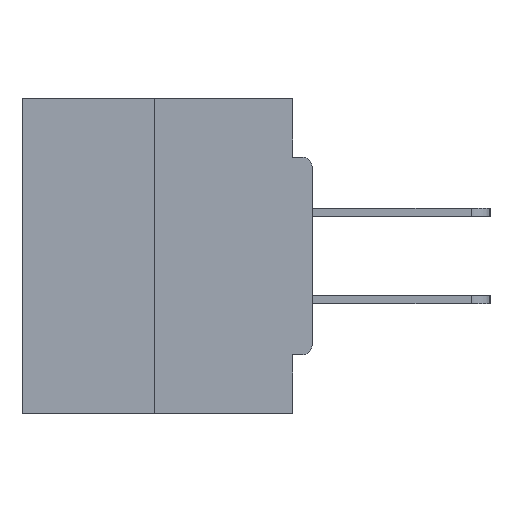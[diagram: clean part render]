
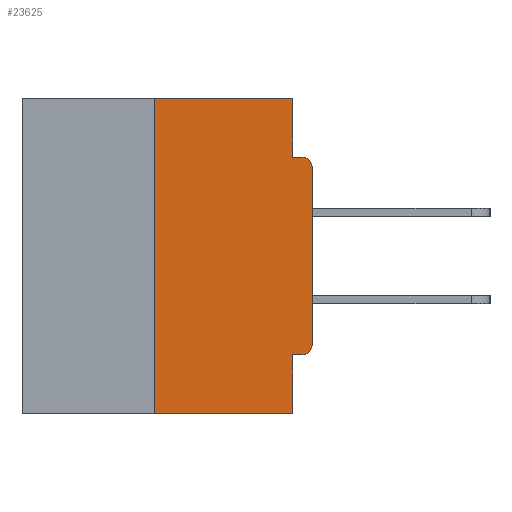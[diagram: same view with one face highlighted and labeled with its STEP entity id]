
A CAD part, left-side view. The second image highlights one B-rep face of the part: STEP entity #23625.
In plain terms, the highlighted planar face has unit normal (-1, 0, 0).
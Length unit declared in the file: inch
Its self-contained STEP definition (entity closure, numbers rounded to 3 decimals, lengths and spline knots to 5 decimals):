
#316 = CARTESIAN_POINT ( 'NONE',  ( 0., 0.25, -0.5 ) ) ;
#655 = VERTEX_POINT ( 'NONE', #3906 ) ;
#974 = LINE ( 'NONE', #31194, #27800 ) ;
#1180 = CARTESIAN_POINT ( 'NONE',  ( 0., 0.031, -0.4065 ) ) ;
#1892 = EDGE_CURVE ( 'NONE', #20515, #12876, #974, .T. ) ;
#2177 = DIRECTION ( 'NONE',  ( -1., 0., 0. ) ) ;
#2508 = CARTESIAN_POINT ( 'NONE',  ( 0., 0.015, -0.1085 ) ) ;
#3137 = LINE ( 'NONE', #16115, #3894 ) ;
#3481 = DIRECTION ( 'NONE',  ( 0., -1., 0. ) ) ;
#3575 = ORIENTED_EDGE ( 'NONE', *, *, #23578, .F. ) ;
#3604 = ORIENTED_EDGE ( 'NONE', *, *, #12128, .F. ) ;
#3894 = VECTOR ( 'NONE', #20548, 39.37008 ) ;
#3906 = CARTESIAN_POINT ( 'NONE',  ( 0., 0.015, -0.0935 ) ) ;
#4278 = DIRECTION ( 'NONE',  ( 0., 0., -1. ) ) ;
#4534 = VERTEX_POINT ( 'NONE', #9252 ) ;
#4629 = DIRECTION ( 'NONE',  ( 0., 0., 1. ) ) ;
#4662 = EDGE_CURVE ( 'NONE', #26802, #655, #10430, .T. ) ;
#4666 = CARTESIAN_POINT ( 'NONE',  ( 0., 0.031, 0. ) ) ;
#5532 = ORIENTED_EDGE ( 'NONE', *, *, #17376, .F. ) ;
#5582 = VERTEX_POINT ( 'NONE', #21843 ) ;
#5725 = CARTESIAN_POINT ( 'NONE',  ( 0., 0., -0.3915 ) ) ;
#5882 = DIRECTION ( 'NONE',  ( 0., 1., 0. ) ) ;
#6043 = DIRECTION ( 'NONE',  ( -1., 0., 0. ) ) ;
#6795 = ORIENTED_EDGE ( 'NONE', *, *, #1892, .F. ) ;
#7691 = EDGE_CURVE ( 'NONE', #27139, #26802, #31581, .T. ) ;
#8728 = CARTESIAN_POINT ( 'NONE',  ( 0., 0.46, 0. ) ) ;
#8793 = CARTESIAN_POINT ( 'NONE',  ( 0., 0.015, -0.4065 ) ) ;
#9252 = CARTESIAN_POINT ( 'NONE',  ( 0., 0.031, -0.0935 ) ) ;
#9364 = LINE ( 'NONE', #19391, #10899 ) ;
#9712 = AXIS2_PLACEMENT_3D ( 'NONE', #23467, #6043, #16069 ) ;
#9913 = CARTESIAN_POINT ( 'NONE',  ( 0., 0.031, 0. ) ) ;
#10430 = CIRCLE ( 'NONE', #30918, 0.015 ) ;
#10448 = CARTESIAN_POINT ( 'NONE',  ( 0., 0.031, -0.5 ) ) ;
#10782 = VERTEX_POINT ( 'NONE', #4666 ) ;
#10874 = VECTOR ( 'NONE', #19602, 39.37008 ) ;
#10899 = VECTOR ( 'NONE', #29411, 39.37008 ) ;
#11346 = CARTESIAN_POINT ( 'NONE',  ( 0., 0.46, 0. ) ) ;
#12128 = EDGE_CURVE ( 'NONE', #23002, #5582, #22257, .T. ) ;
#12876 = VERTEX_POINT ( 'NONE', #1180 ) ;
#16069 = DIRECTION ( 'NONE',  ( 0., 0., -1. ) ) ;
#16115 = CARTESIAN_POINT ( 'NONE',  ( 0., 0., -0.0935 ) ) ;
#16606 = VECTOR ( 'NONE', #3481, 39.37008 ) ;
#17376 = EDGE_CURVE ( 'NONE', #5582, #10782, #19076, .T. ) ;
#17404 = ORIENTED_EDGE ( 'NONE', *, *, #4662, .T. ) ;
#18247 = ORIENTED_EDGE ( 'NONE', *, *, #7691, .T. ) ;
#18555 = EDGE_LOOP ( 'NONE', ( #5532, #3604, #29578, #3575, #6795, #25475, #18247, #17404, #24689, #27252 ) ) ;
#18741 = EDGE_CURVE ( 'NONE', #20515, #27139, #23890, .T. ) ;
#18760 = PLANE ( 'NONE',  #28768 ) ;
#18796 = LINE ( 'NONE', #19420, #30150 ) ;
#19076 = LINE ( 'NONE', #8728, #16606 ) ;
#19230 = FACE_OUTER_BOUND ( 'NONE', #18555, .T. ) ;
#19391 = CARTESIAN_POINT ( 'NONE',  ( 0., 0.031, -0.5 ) ) ;
#19420 = CARTESIAN_POINT ( 'NONE',  ( 0., 0.46, -0.5 ) ) ;
#19602 = DIRECTION ( 'NONE',  ( 0., 0., -1. ) ) ;
#20515 = VERTEX_POINT ( 'NONE', #8793 ) ;
#20548 = DIRECTION ( 'NONE',  ( 0., -1., 0. ) ) ;
#20625 = EDGE_CURVE ( 'NONE', #10782, #4534, #32255, .T. ) ;
#21574 = CARTESIAN_POINT ( 'NONE',  ( 0., 0., 0. ) ) ;
#21580 = DIRECTION ( 'NONE',  ( 0., -1., 0. ) ) ;
#21843 = CARTESIAN_POINT ( 'NONE',  ( 0., 0.25, 0. ) ) ;
#22018 = DIRECTION ( 'NONE',  ( 1., 0., 0. ) ) ;
#22234 = VECTOR ( 'NONE', #31807, 39.37008 ) ;
#22257 = LINE ( 'NONE', #32276, #22234 ) ;
#23002 = VERTEX_POINT ( 'NONE', #316 ) ;
#23467 = CARTESIAN_POINT ( 'NONE',  ( 0., 0.015, -0.3915 ) ) ;
#23578 = EDGE_CURVE ( 'NONE', #12876, #32240, #9364, .T. ) ;
#23625 = ADVANCED_FACE ( 'NONE', ( #19230 ), #18760, .F. ) ;
#23663 = CARTESIAN_POINT ( 'NONE',  ( 0., 0., -0.1085 ) ) ;
#23890 = CIRCLE ( 'NONE', #9712, 0.015 ) ;
#24689 = ORIENTED_EDGE ( 'NONE', *, *, #28643, .F. ) ;
#24690 = DIRECTION ( 'NONE',  ( 0., 0., -1. ) ) ;
#25475 = ORIENTED_EDGE ( 'NONE', *, *, #18741, .T. ) ;
#26802 = VERTEX_POINT ( 'NONE', #23663 ) ;
#27139 = VERTEX_POINT ( 'NONE', #5725 ) ;
#27252 = ORIENTED_EDGE ( 'NONE', *, *, #20625, .F. ) ;
#27800 = VECTOR ( 'NONE', #5882, 39.37008 ) ;
#28643 = EDGE_CURVE ( 'NONE', #4534, #655, #3137, .T. ) ;
#28768 = AXIS2_PLACEMENT_3D ( 'NONE', #11346, #22018, #4278 ) ;
#29411 = DIRECTION ( 'NONE',  ( 0., 0., -1. ) ) ;
#29578 = ORIENTED_EDGE ( 'NONE', *, *, #29597, .T. ) ;
#29597 = EDGE_CURVE ( 'NONE', #23002, #32240, #18796, .T. ) ;
#30040 = VECTOR ( 'NONE', #4629, 39.37008 ) ;
#30150 = VECTOR ( 'NONE', #21580, 39.37008 ) ;
#30918 = AXIS2_PLACEMENT_3D ( 'NONE', #2508, #2177, #24690 ) ;
#31194 = CARTESIAN_POINT ( 'NONE',  ( 0., 0., -0.4065 ) ) ;
#31581 = LINE ( 'NONE', #21574, #30040 ) ;
#31807 = DIRECTION ( 'NONE',  ( 0., 0., 1. ) ) ;
#32240 = VERTEX_POINT ( 'NONE', #10448 ) ;
#32255 = LINE ( 'NONE', #9913, #10874 ) ;
#32276 = CARTESIAN_POINT ( 'NONE',  ( 0., 0.25, 0. ) ) ;
